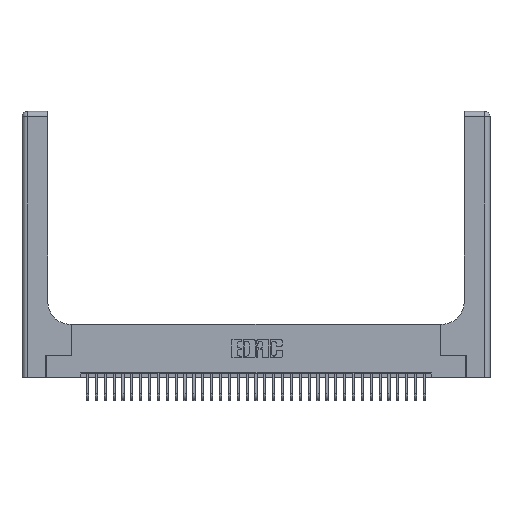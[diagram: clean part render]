
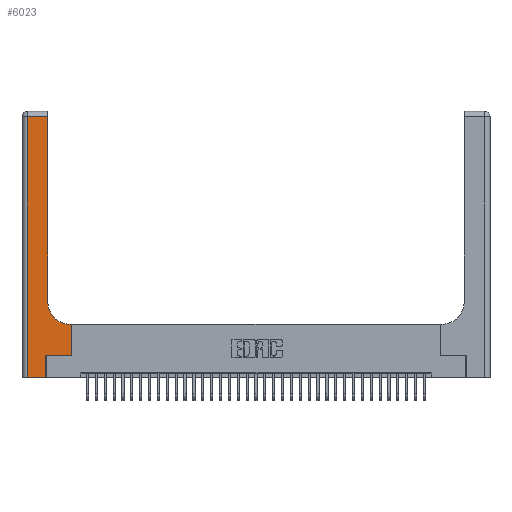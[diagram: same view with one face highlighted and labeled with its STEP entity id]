
A CAD part, top view. The second image highlights one B-rep face of the part: STEP entity #6023.
In plain terms, the highlighted planar face has unit normal (0, 0, 1).
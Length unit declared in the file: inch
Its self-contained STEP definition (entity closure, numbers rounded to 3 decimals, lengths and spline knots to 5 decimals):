
#1106 = LINE ( 'NONE', #10881, #22715 ) ;
#1187 = DIRECTION ( 'NONE',  ( -1., 0., 0. ) ) ;
#1562 = CARTESIAN_POINT ( 'NONE',  ( 0.5585, 0.6, 0.37 ) ) ;
#1836 = CARTESIAN_POINT ( 'NONE',  ( 0.2915, 3., 0.37 ) ) ;
#2097 = VERTEX_POINT ( 'NONE', #19014 ) ;
#2374 = ORIENTED_EDGE ( 'NONE', *, *, #25611, .T. ) ;
#2737 = EDGE_CURVE ( 'NONE', #7874, #26865, #33673, .T. ) ;
#3434 = CARTESIAN_POINT ( 'NONE',  ( 0.2915, 0.85, 0.37 ) ) ;
#3642 = VECTOR ( 'NONE', #7533, 39.37008 ) ;
#4282 = DIRECTION ( 'NONE',  ( -1., 0., 0. ) ) ;
#4597 = VECTOR ( 'NONE', #4282, 39.37008 ) ;
#4796 = VERTEX_POINT ( 'NONE', #33760 ) ;
#5484 = VECTOR ( 'NONE', #7350, 39.37008 ) ;
#5656 = CARTESIAN_POINT ( 'NONE',  ( 0.5415, 0.85, 0.37 ) ) ;
#6023 = ADVANCED_FACE ( 'NONE', ( #8753 ), #14615, .F. ) ;
#6359 = CARTESIAN_POINT ( 'NONE',  ( 0., 0., 0.37 ) ) ;
#6475 = CIRCLE ( 'NONE', #19262, 0.25 ) ;
#7350 = DIRECTION ( 'NONE',  ( 0., 1., 0. ) ) ;
#7533 = DIRECTION ( 'NONE',  ( 1., 0., 0. ) ) ;
#7874 = VERTEX_POINT ( 'NONE', #15384 ) ;
#8397 = DIRECTION ( 'NONE',  ( 1., 0., 0. ) ) ;
#8753 = FACE_OUTER_BOUND ( 'NONE', #15162, .T. ) ;
#9319 = CARTESIAN_POINT ( 'NONE',  ( 0., 3., 0.37 ) ) ;
#9698 = EDGE_CURVE ( 'NONE', #17214, #4796, #31279, .T. ) ;
#10066 = DIRECTION ( 'NONE',  ( 0., 1., 0. ) ) ;
#10881 = CARTESIAN_POINT ( 'NONE',  ( 0.06, 3., 0.37 ) ) ;
#11350 = VECTOR ( 'NONE', #10066, 39.37008 ) ;
#11712 = LINE ( 'NONE', #23706, #3642 ) ;
#11819 = LINE ( 'NONE', #23183, #4597 ) ;
#12269 = VECTOR ( 'NONE', #17784, 39.37008 ) ;
#12329 = ORIENTED_EDGE ( 'NONE', *, *, #31343, .T. ) ;
#13550 = CARTESIAN_POINT ( 'NONE',  ( 0.06, 2.94, 0.37 ) ) ;
#13692 = DIRECTION ( 'NONE',  ( -1., 0., 0. ) ) ;
#14615 = PLANE ( 'NONE',  #25326 ) ;
#14660 = VERTEX_POINT ( 'NONE', #3434 ) ;
#15089 = CARTESIAN_POINT ( 'NONE',  ( 0.5585, 0.25, 0.37 ) ) ;
#15162 = EDGE_LOOP ( 'NONE', ( #2374, #26966, #29511, #32906, #21949, #25312, #15208, #29586, #12329 ) ) ;
#15208 = ORIENTED_EDGE ( 'NONE', *, *, #19366, .T. ) ;
#15384 = CARTESIAN_POINT ( 'NONE',  ( 0.06, 0., 0.37 ) ) ;
#15400 = EDGE_CURVE ( 'NONE', #2097, #19325, #11712, .T. ) ;
#16109 = VECTOR ( 'NONE', #13692, 39.37008 ) ;
#17081 = DIRECTION ( 'NONE',  ( 1., 0., 0. ) ) ;
#17214 = VERTEX_POINT ( 'NONE', #1562 ) ;
#17426 = DIRECTION ( 'NONE',  ( 0., 0., -1. ) ) ;
#17517 = CARTESIAN_POINT ( 'NONE',  ( 0.2915, 2.94, 0.37 ) ) ;
#17784 = DIRECTION ( 'NONE',  ( 0., 1., 0. ) ) ;
#18157 = CARTESIAN_POINT ( 'NONE',  ( 0.269, 0., 0.37 ) ) ;
#19014 = CARTESIAN_POINT ( 'NONE',  ( 0.269, 0.25, 0.37 ) ) ;
#19262 = AXIS2_PLACEMENT_3D ( 'NONE', #5656, #24535, #8397 ) ;
#19325 = VERTEX_POINT ( 'NONE', #22983 ) ;
#19345 = LINE ( 'NONE', #18157, #11350 ) ;
#19366 = EDGE_CURVE ( 'NONE', #19325, #17214, #26566, .T. ) ;
#19602 = VERTEX_POINT ( 'NONE', #13550 ) ;
#19683 = CARTESIAN_POINT ( 'NONE',  ( 0.269, 0., 0.37 ) ) ;
#20328 = EDGE_CURVE ( 'NONE', #30294, #19602, #11819, .T. ) ;
#20988 = EDGE_CURVE ( 'NONE', #26865, #2097, #19345, .T. ) ;
#21949 = ORIENTED_EDGE ( 'NONE', *, *, #20988, .T. ) ;
#22715 = VECTOR ( 'NONE', #32419, 39.37008 ) ;
#22983 = CARTESIAN_POINT ( 'NONE',  ( 0.5585, 0.25, 0.37 ) ) ;
#23183 = CARTESIAN_POINT ( 'NONE',  ( 0., 2.94, 0.37 ) ) ;
#23706 = CARTESIAN_POINT ( 'NONE',  ( 0.269, 0.25, 0.37 ) ) ;
#24535 = DIRECTION ( 'NONE',  ( 0., 0., -1. ) ) ;
#25312 = ORIENTED_EDGE ( 'NONE', *, *, #15400, .T. ) ;
#25326 = AXIS2_PLACEMENT_3D ( 'NONE', #9319, #17426, #1187 ) ;
#25611 = EDGE_CURVE ( 'NONE', #14660, #30294, #27004, .T. ) ;
#26491 = VECTOR ( 'NONE', #17081, 39.37008 ) ;
#26566 = LINE ( 'NONE', #15089, #12269 ) ;
#26689 = EDGE_CURVE ( 'NONE', #19602, #7874, #1106, .T. ) ;
#26865 = VERTEX_POINT ( 'NONE', #19683 ) ;
#26966 = ORIENTED_EDGE ( 'NONE', *, *, #20328, .T. ) ;
#27004 = LINE ( 'NONE', #1836, #5484 ) ;
#27099 = CARTESIAN_POINT ( 'NONE',  ( 0.2915, 0.6, 0.37 ) ) ;
#29511 = ORIENTED_EDGE ( 'NONE', *, *, #26689, .T. ) ;
#29586 = ORIENTED_EDGE ( 'NONE', *, *, #9698, .T. ) ;
#30294 = VERTEX_POINT ( 'NONE', #17517 ) ;
#31279 = LINE ( 'NONE', #27099, #16109 ) ;
#31343 = EDGE_CURVE ( 'NONE', #4796, #14660, #6475, .T. ) ;
#32419 = DIRECTION ( 'NONE',  ( 0., -1., 0. ) ) ;
#32906 = ORIENTED_EDGE ( 'NONE', *, *, #2737, .T. ) ;
#33673 = LINE ( 'NONE', #6359, #26491 ) ;
#33760 = CARTESIAN_POINT ( 'NONE',  ( 0.5415, 0.6, 0.37 ) ) ;
